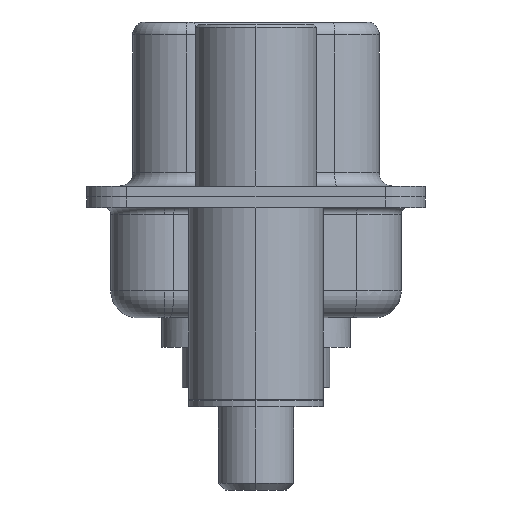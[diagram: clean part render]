
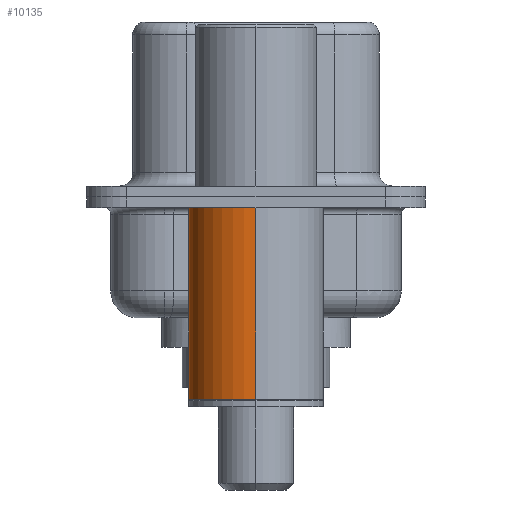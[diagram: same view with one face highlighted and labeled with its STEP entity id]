
A CAD part, left-side view. The second image highlights one B-rep face of the part: STEP entity #10135.
In plain terms, the highlighted cylindrical face has radius 2.5 mm (diameter 5 mm), a partial arc.
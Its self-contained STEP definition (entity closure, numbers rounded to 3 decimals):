
#430 = DIRECTION ( 'NONE',  ( 0., 0., 1. ) ) ;
#649 = CIRCLE ( 'NONE', #11343, 2.5 ) ;
#1369 = CARTESIAN_POINT ( 'NONE',  ( 0., 0., -0.4 ) ) ;
#1408 = CARTESIAN_POINT ( 'NONE',  ( 0., 0., -7.525 ) ) ;
#2077 = CARTESIAN_POINT ( 'NONE',  ( 2.5, 0., -0.4 ) ) ;
#2614 = VERTEX_POINT ( 'NONE', #10589 ) ;
#2795 = CARTESIAN_POINT ( 'NONE',  ( -2.5, 0., 0.581 ) ) ;
#2803 = DIRECTION ( 'NONE',  ( 1., 0., 0. ) ) ;
#3016 = CIRCLE ( 'NONE', #16706, 2.5 ) ;
#4689 = VERTEX_POINT ( 'NONE', #6922 ) ;
#4724 = CYLINDRICAL_SURFACE ( 'NONE', #5441, 2.5 ) ;
#5021 = DIRECTION ( 'NONE',  ( 1., 0., 0. ) ) ;
#5229 = EDGE_CURVE ( 'NONE', #2614, #4689, #17307, .T. ) ;
#5441 = AXIS2_PLACEMENT_3D ( 'NONE', #14375, #15769, #15701 ) ;
#5516 = ORIENTED_EDGE ( 'NONE', *, *, #16392, .F. ) ;
#5657 = DIRECTION ( 'NONE',  ( 0., 0., 1. ) ) ;
#5660 = ORIENTED_EDGE ( 'NONE', *, *, #16284, .T. ) ;
#6170 = LINE ( 'NONE', #13587, #16831 ) ;
#6218 = DIRECTION ( 'NONE',  ( 0., 0., 1. ) ) ;
#6465 = EDGE_CURVE ( 'NONE', #15326, #4689, #3016, .T. ) ;
#6557 = ORIENTED_EDGE ( 'NONE', *, *, #6465, .F. ) ;
#6922 = CARTESIAN_POINT ( 'NONE',  ( -2.5, 0., -0.4 ) ) ;
#10135 = ADVANCED_FACE ( 'NONE', ( #15795 ), #4724, .T. ) ;
#10165 = VECTOR ( 'NONE', #430, 1000. ) ;
#10589 = CARTESIAN_POINT ( 'NONE',  ( -2.5, 0., -7.525 ) ) ;
#10797 = DIRECTION ( 'NONE',  ( 0., 0., 1. ) ) ;
#11263 = VERTEX_POINT ( 'NONE', #15291 ) ;
#11343 = AXIS2_PLACEMENT_3D ( 'NONE', #1408, #10797, #2803 ) ;
#13587 = CARTESIAN_POINT ( 'NONE',  ( 2.5, 0., 0.581 ) ) ;
#14375 = CARTESIAN_POINT ( 'NONE',  ( 0., 0., 0.581 ) ) ;
#14564 = EDGE_LOOP ( 'NONE', ( #5660, #16034, #6557, #5516 ) ) ;
#15291 = CARTESIAN_POINT ( 'NONE',  ( 2.5, 0., -7.525 ) ) ;
#15326 = VERTEX_POINT ( 'NONE', #2077 ) ;
#15701 = DIRECTION ( 'NONE',  ( 1., 0., 0. ) ) ;
#15769 = DIRECTION ( 'NONE',  ( 0., 0., 1. ) ) ;
#15795 = FACE_OUTER_BOUND ( 'NONE', #14564, .T. ) ;
#16034 = ORIENTED_EDGE ( 'NONE', *, *, #5229, .T. ) ;
#16284 = EDGE_CURVE ( 'NONE', #11263, #2614, #649, .T. ) ;
#16392 = EDGE_CURVE ( 'NONE', #11263, #15326, #6170, .T. ) ;
#16706 = AXIS2_PLACEMENT_3D ( 'NONE', #1369, #6218, #5021 ) ;
#16831 = VECTOR ( 'NONE', #5657, 1000. ) ;
#17307 = LINE ( 'NONE', #2795, #10165 ) ;
